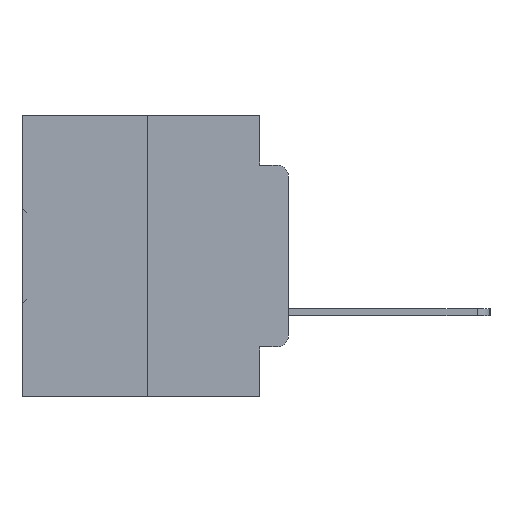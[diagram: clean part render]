
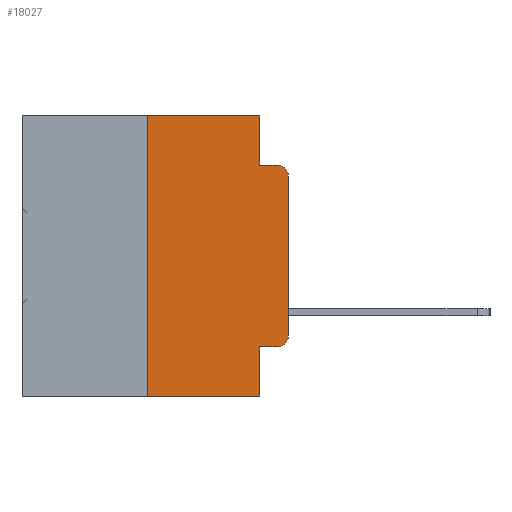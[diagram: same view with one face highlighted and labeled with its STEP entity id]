
A CAD part, left-side view. The second image highlights one B-rep face of the part: STEP entity #18027.
In plain terms, the highlighted planar face has unit normal (-1, 0, 0).
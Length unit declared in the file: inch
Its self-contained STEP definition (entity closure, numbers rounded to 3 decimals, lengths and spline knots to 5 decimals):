
#694 = EDGE_CURVE ( 'NONE', #12106, #27278, #15959, .T. ) ;
#776 = DIRECTION ( 'NONE',  ( 0., 0., -1. ) ) ;
#1523 = CARTESIAN_POINT ( 'NONE',  ( 0., 0., -0.3915 ) ) ;
#1526 = VERTEX_POINT ( 'NONE', #11487 ) ;
#2104 = ORIENTED_EDGE ( 'NONE', *, *, #694, .T. ) ;
#2198 = LINE ( 'NONE', #2587, #28997 ) ;
#2573 = VECTOR ( 'NONE', #15377, 39.37008 ) ;
#2587 = CARTESIAN_POINT ( 'NONE',  ( 0., 0.473, -0.5 ) ) ;
#2701 = DIRECTION ( 'NONE',  ( 0., -1., 0. ) ) ;
#2992 = VERTEX_POINT ( 'NONE', #26158 ) ;
#3981 = CIRCLE ( 'NONE', #6569, 0.02 ) ;
#6569 = AXIS2_PLACEMENT_3D ( 'NONE', #7958, #26057, #10687 ) ;
#6995 = VERTEX_POINT ( 'NONE', #8540 ) ;
#7772 = DIRECTION ( 'NONE',  ( 0., 0., -1. ) ) ;
#7958 = CARTESIAN_POINT ( 'NONE',  ( 0., 0.02, -0.3915 ) ) ;
#8486 = ORIENTED_EDGE ( 'NONE', *, *, #31925, .F. ) ;
#8540 = CARTESIAN_POINT ( 'NONE',  ( 0., 0.051, -0.0885 ) ) ;
#8840 = VERTEX_POINT ( 'NONE', #16256 ) ;
#9684 = AXIS2_PLACEMENT_3D ( 'NONE', #11455, #16699, #776 ) ;
#9752 = LINE ( 'NONE', #17909, #2573 ) ;
#10191 = VECTOR ( 'NONE', #25526, 39.37008 ) ;
#10208 = AXIS2_PLACEMENT_3D ( 'NONE', #11699, #11736, #13193 ) ;
#10678 = DIRECTION ( 'NONE',  ( 0., 0., -1. ) ) ;
#10687 = DIRECTION ( 'NONE',  ( 0., 0., -1. ) ) ;
#10757 = LINE ( 'NONE', #14380, #30290 ) ;
#11023 = LINE ( 'NONE', #15256, #10191 ) ;
#11038 = EDGE_CURVE ( 'NONE', #25968, #29120, #3981, .T. ) ;
#11384 = DIRECTION ( 'NONE',  ( 0., 0., 1. ) ) ;
#11455 = CARTESIAN_POINT ( 'NONE',  ( 0., 0.473, 0. ) ) ;
#11487 = CARTESIAN_POINT ( 'NONE',  ( 0., 0.051, -0.4115 ) ) ;
#11699 = CARTESIAN_POINT ( 'NONE',  ( 0., 0.02, -0.1085 ) ) ;
#11736 = DIRECTION ( 'NONE',  ( -1., 0., 0. ) ) ;
#12106 = VERTEX_POINT ( 'NONE', #17459 ) ;
#12377 = EDGE_CURVE ( 'NONE', #28630, #2992, #2198, .T. ) ;
#12765 = EDGE_CURVE ( 'NONE', #1526, #25968, #11023, .T. ) ;
#13105 = CARTESIAN_POINT ( 'NONE',  ( 0., 0.051, 0. ) ) ;
#13193 = DIRECTION ( 'NONE',  ( 0., 0., -1. ) ) ;
#13490 = LINE ( 'NONE', #26049, #27105 ) ;
#13665 = CARTESIAN_POINT ( 'NONE',  ( 0., 0., 0. ) ) ;
#13840 = VERTEX_POINT ( 'NONE', #14381 ) ;
#14035 = PLANE ( 'NONE',  #9684 ) ;
#14380 = CARTESIAN_POINT ( 'NONE',  ( 0., 0.473, 0. ) ) ;
#14381 = CARTESIAN_POINT ( 'NONE',  ( 0., 0.25, 0. ) ) ;
#15065 = ORIENTED_EDGE ( 'NONE', *, *, #12377, .T. ) ;
#15179 = VECTOR ( 'NONE', #7772, 39.37008 ) ;
#15256 = CARTESIAN_POINT ( 'NONE',  ( 0., 0.051, -0.4115 ) ) ;
#15377 = DIRECTION ( 'NONE',  ( 0., -1., 0. ) ) ;
#15959 = CIRCLE ( 'NONE', #10208, 0.02 ) ;
#16013 = LINE ( 'NONE', #13105, #15179 ) ;
#16256 = CARTESIAN_POINT ( 'NONE',  ( 0., 0.051, 0. ) ) ;
#16699 = DIRECTION ( 'NONE',  ( 1., 0., 0. ) ) ;
#16725 = EDGE_CURVE ( 'NONE', #29120, #12106, #31939, .T. ) ;
#17365 = EDGE_CURVE ( 'NONE', #28630, #13840, #31486, .T. ) ;
#17459 = CARTESIAN_POINT ( 'NONE',  ( 0., 0., -0.1085 ) ) ;
#17634 = ORIENTED_EDGE ( 'NONE', *, *, #11038, .T. ) ;
#17909 = CARTESIAN_POINT ( 'NONE',  ( 0., 0.051, -0.0885 ) ) ;
#18027 = ADVANCED_FACE ( 'NONE', ( #25203 ), #14035, .F. ) ;
#19760 = EDGE_CURVE ( 'NONE', #1526, #2992, #13490, .T. ) ;
#20818 = EDGE_CURVE ( 'NONE', #8840, #6995, #16013, .T. ) ;
#22510 = EDGE_CURVE ( 'NONE', #6995, #27278, #9752, .T. ) ;
#22815 = ORIENTED_EDGE ( 'NONE', *, *, #22510, .F. ) ;
#24000 = DIRECTION ( 'NONE',  ( 0., 0., 1. ) ) ;
#24379 = EDGE_LOOP ( 'NONE', ( #30569, #2104, #22815, #27870, #8486, #31419, #15065, #25698, #26575, #17634 ) ) ;
#24885 = CARTESIAN_POINT ( 'NONE',  ( 0., 0.02, -0.0885 ) ) ;
#25203 = FACE_OUTER_BOUND ( 'NONE', #24379, .T. ) ;
#25526 = DIRECTION ( 'NONE',  ( 0., -1., 0. ) ) ;
#25698 = ORIENTED_EDGE ( 'NONE', *, *, #19760, .F. ) ;
#25968 = VERTEX_POINT ( 'NONE', #32245 ) ;
#26049 = CARTESIAN_POINT ( 'NONE',  ( 0., 0.051, 0. ) ) ;
#26057 = DIRECTION ( 'NONE',  ( -1., 0., 0. ) ) ;
#26158 = CARTESIAN_POINT ( 'NONE',  ( 0., 0.051, -0.5 ) ) ;
#26424 = VECTOR ( 'NONE', #11384, 39.37008 ) ;
#26575 = ORIENTED_EDGE ( 'NONE', *, *, #12765, .T. ) ;
#26710 = CARTESIAN_POINT ( 'NONE',  ( 0., 0.25, 0. ) ) ;
#27105 = VECTOR ( 'NONE', #10678, 39.37008 ) ;
#27117 = DIRECTION ( 'NONE',  ( 0., -1., 0. ) ) ;
#27278 = VERTEX_POINT ( 'NONE', #24885 ) ;
#27870 = ORIENTED_EDGE ( 'NONE', *, *, #20818, .F. ) ;
#28062 = CARTESIAN_POINT ( 'NONE',  ( 0., 0.25, -0.5 ) ) ;
#28630 = VERTEX_POINT ( 'NONE', #28062 ) ;
#28997 = VECTOR ( 'NONE', #2701, 39.37008 ) ;
#29120 = VERTEX_POINT ( 'NONE', #1523 ) ;
#30290 = VECTOR ( 'NONE', #27117, 39.37008 ) ;
#30359 = VECTOR ( 'NONE', #24000, 39.37008 ) ;
#30569 = ORIENTED_EDGE ( 'NONE', *, *, #16725, .T. ) ;
#31419 = ORIENTED_EDGE ( 'NONE', *, *, #17365, .F. ) ;
#31486 = LINE ( 'NONE', #26710, #26424 ) ;
#31925 = EDGE_CURVE ( 'NONE', #13840, #8840, #10757, .T. ) ;
#31939 = LINE ( 'NONE', #13665, #30359 ) ;
#32245 = CARTESIAN_POINT ( 'NONE',  ( 0., 0.02, -0.4115 ) ) ;
